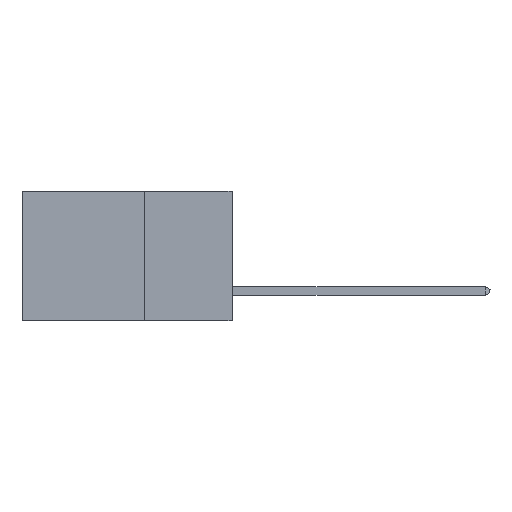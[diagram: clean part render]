
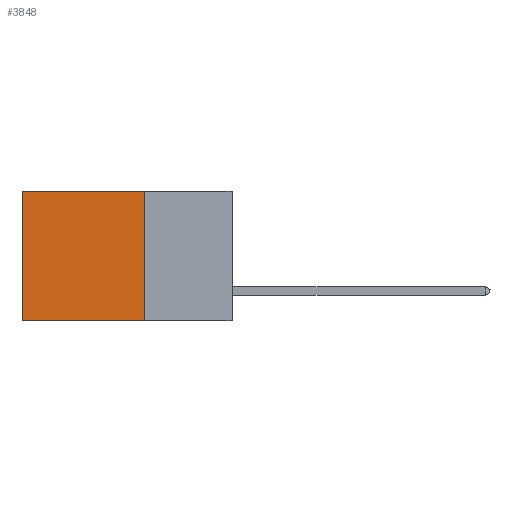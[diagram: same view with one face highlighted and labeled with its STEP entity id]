
A CAD part, left-side view. The second image highlights one B-rep face of the part: STEP entity #3848.
In plain terms, the highlighted planar face has unit normal (-1, 0, 0).
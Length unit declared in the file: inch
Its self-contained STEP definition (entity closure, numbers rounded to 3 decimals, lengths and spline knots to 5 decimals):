
#229 = EDGE_CURVE ( 'NONE', #16419, #18578, #10199, .T. ) ;
#364 = DIRECTION ( 'NONE',  ( 0., 0., -1. ) ) ;
#1587 = CARTESIAN_POINT ( 'NONE',  ( 0.2875, 0.25, -0.37 ) ) ;
#2090 = PLANE ( 'NONE',  #14387 ) ;
#2669 = VERTEX_POINT ( 'NONE', #18371 ) ;
#2963 = CARTESIAN_POINT ( 'NONE',  ( 0.2875, 0.6, 0. ) ) ;
#3046 = ORIENTED_EDGE ( 'NONE', *, *, #17768, .F. ) ;
#3848 = ADVANCED_FACE ( 'NONE', ( #8724 ), #2090, .F. ) ;
#4182 = CARTESIAN_POINT ( 'NONE',  ( 0.2875, 0.25, 0. ) ) ;
#5681 = CARTESIAN_POINT ( 'NONE',  ( 0.2875, 0.25, 0. ) ) ;
#5817 = CARTESIAN_POINT ( 'NONE',  ( 0.2875, 0.6, 0. ) ) ;
#7120 = VERTEX_POINT ( 'NONE', #9209 ) ;
#7168 = ORIENTED_EDGE ( 'NONE', *, *, #229, .T. ) ;
#7220 = LINE ( 'NONE', #1587, #15717 ) ;
#7721 = ORIENTED_EDGE ( 'NONE', *, *, #7918, .F. ) ;
#7918 = EDGE_CURVE ( 'NONE', #7120, #2669, #9944, .T. ) ;
#8724 = FACE_OUTER_BOUND ( 'NONE', #10735, .T. ) ;
#9209 = CARTESIAN_POINT ( 'NONE',  ( 0.2875, 0.25, 0. ) ) ;
#9944 = LINE ( 'NONE', #5681, #11302 ) ;
#10199 = LINE ( 'NONE', #2963, #16006 ) ;
#10227 = DIRECTION ( 'NONE',  ( 0., 0., -1. ) ) ;
#10621 = CARTESIAN_POINT ( 'NONE',  ( 0.2875, 0.6, -0.37 ) ) ;
#10735 = EDGE_LOOP ( 'NONE', ( #7168, #3046, #7721, #13958 ) ) ;
#11302 = VECTOR ( 'NONE', #364, 39.37008 ) ;
#12244 = DIRECTION ( 'NONE',  ( 1., 0., 0. ) ) ;
#13019 = VECTOR ( 'NONE', #14265, 39.37008 ) ;
#13073 = DIRECTION ( 'NONE',  ( 0., 1., 0. ) ) ;
#13958 = ORIENTED_EDGE ( 'NONE', *, *, #17677, .T. ) ;
#14265 = DIRECTION ( 'NONE',  ( 0., 1., 0. ) ) ;
#14387 = AXIS2_PLACEMENT_3D ( 'NONE', #14863, #12244, #16370 ) ;
#14863 = CARTESIAN_POINT ( 'NONE',  ( 0.2875, 0.25, 0. ) ) ;
#15717 = VECTOR ( 'NONE', #13073, 39.37008 ) ;
#16006 = VECTOR ( 'NONE', #10227, 39.37008 ) ;
#16370 = DIRECTION ( 'NONE',  ( 0., 0., -1. ) ) ;
#16419 = VERTEX_POINT ( 'NONE', #5817 ) ;
#16828 = LINE ( 'NONE', #4182, #13019 ) ;
#17677 = EDGE_CURVE ( 'NONE', #7120, #16419, #16828, .T. ) ;
#17768 = EDGE_CURVE ( 'NONE', #2669, #18578, #7220, .T. ) ;
#18371 = CARTESIAN_POINT ( 'NONE',  ( 0.2875, 0.25, -0.37 ) ) ;
#18578 = VERTEX_POINT ( 'NONE', #10621 ) ;
